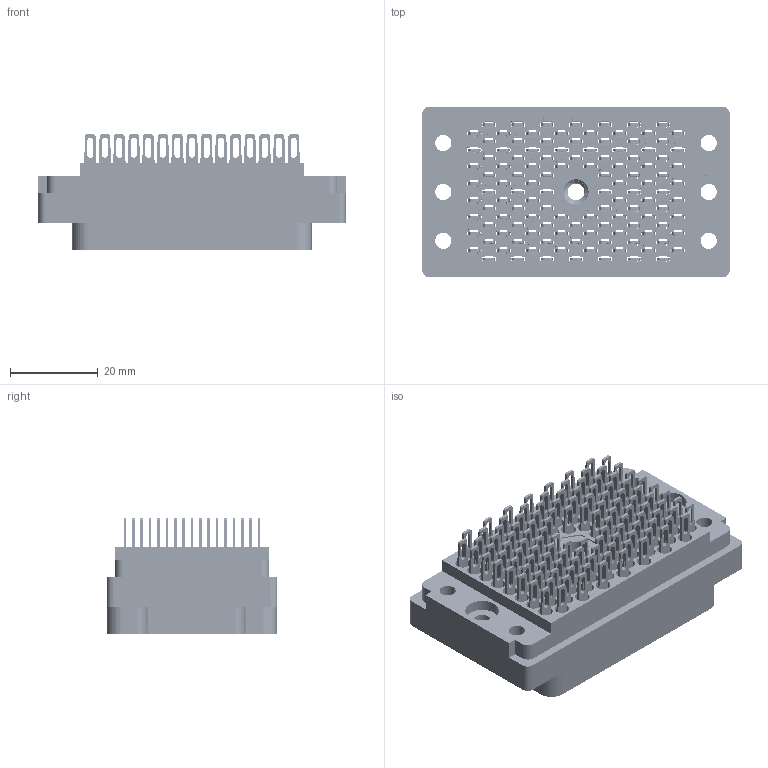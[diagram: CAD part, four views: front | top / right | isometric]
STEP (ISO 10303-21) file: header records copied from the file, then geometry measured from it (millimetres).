
FILE_DESCRIPTION (( 'STEP AP203' ), '1' );
FILE_NAME ('516-120-500-306.STEP', '2020-03-11T02:34:35', ( '' ), ( '' ), 'SwSTEP 2.0', 'SolidWorks 2016', '' );
FILE_SCHEMA (( 'CONFIG_CONTROL_DESIGN' ));
Length unit declared in the file: inch
Products named in the file (4): 516-252-095-100; 516-292-001_500 Contact; 516-120-500-306; 516 Plug Insulator_120
Assembly tree (122 placements, depth 2):
  516-120-500-306
    516 Plug Insulator_120
    516-292-001_500 Contact  x120
    516-252-095-100
Bounding box: 69.85 x 38.73 x 26.26 mm (x, y, z)
Volume: 23930.1 mm3; surface area: 49185.9 mm2
Topology: 122 solids, 122 shells, 11549 faces, 33621 edges, 22331 vertices
Faces by surface type: plane 6970, cylinder 3841, bspline 726, cone 12
Entity records: 90613 total; most frequent: CARTESIAN_POINT 17317, ORIENTED_EDGE 14882, DIRECTION 14322, EDGE_CURVE 7441, VECTOR 5632, LINE 5632, VERTEX_POINT 4957, AXIS2_PLACEMENT_3D 4345
